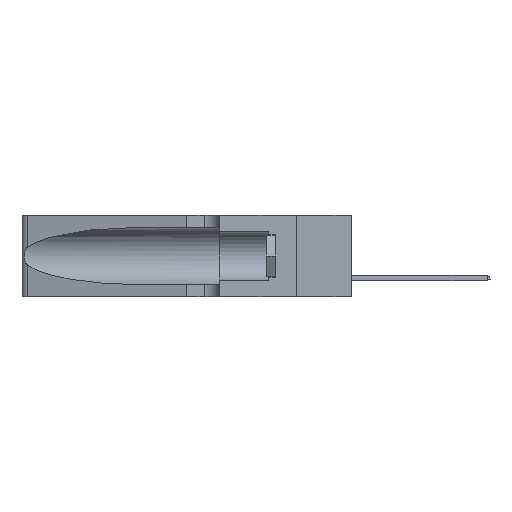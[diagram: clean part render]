
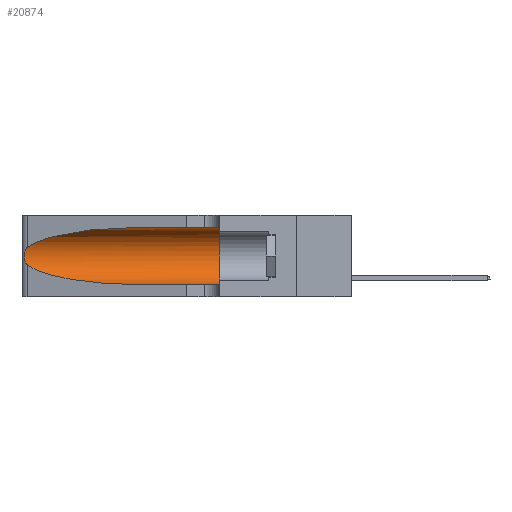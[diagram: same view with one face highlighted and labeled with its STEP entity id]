
A CAD part, left-side view. The second image highlights one B-rep face of the part: STEP entity #20874.
In plain terms, the highlighted cylindrical face has radius 3.308 mm (diameter 6.617 mm), a partial arc.
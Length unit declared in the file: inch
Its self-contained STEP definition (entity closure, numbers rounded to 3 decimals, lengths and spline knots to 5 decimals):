
#215 = CARTESIAN_POINT ( 'NONE',  ( 0.18966, 0.96281, 0.31525 ) ) ;
#1623 = VECTOR ( 'NONE', #15362, 39.37008 ) ;
#1929 = CARTESIAN_POINT ( 'NONE',  ( 0.25487, 1.22718, 0.14631 ) ) ;
#2081 = DIRECTION ( 'NONE',  ( 0., -1., 0. ) ) ;
#2461 = EDGE_CURVE ( 'NONE', #21685, #13691, #21260, .T. ) ;
#2652 = CARTESIAN_POINT ( 'NONE',  ( 0.1305, 0.72297, 0.05475 ) ) ;
#3155 = EDGE_CURVE ( 'NONE', #7632, #14340, #14061, .T. ) ;
#3199 = CARTESIAN_POINT ( 'NONE',  ( 0.25487, 1.22718, 0.14631 ) ) ;
#3279 = EDGE_CURVE ( 'NONE', #3822, #7632, #8387, .T. ) ;
#3552 = CARTESIAN_POINT ( 'NONE',  ( 0.25555, 1.22993, 0.14849 ) ) ;
#3650 = CYLINDRICAL_SURFACE ( 'NONE', #13707, 0.13025 ) ;
#3729 = CARTESIAN_POINT ( 'NONE',  ( 0.25487, 1.22718, 0.14631 ) ) ;
#3822 = VERTEX_POINT ( 'NONE', #19467 ) ;
#3871 = CARTESIAN_POINT ( 'NONE',  ( 0.1305, 0.35, 0.31525 ) ) ;
#4050 = ORIENTED_EDGE ( 'NONE', *, *, #19851, .F. ) ;
#4903 = CARTESIAN_POINT ( 'NONE',  ( 0.18966, 0.96281, 0.05475 ) ) ;
#5049 = CARTESIAN_POINT ( 'NONE',  ( 0.1305, 0.72297, 0.05475 ) ) ;
#5426 = EDGE_LOOP ( 'NONE', ( #5481, #6778, #6812, #5883, #4050, #7863 ) ) ;
#5481 = ORIENTED_EDGE ( 'NONE', *, *, #12679, .T. ) ;
#5562 = CARTESIAN_POINT ( 'NONE',  ( 0.1305, 1.61858, 0.05475 ) ) ;
#5883 = ORIENTED_EDGE ( 'NONE', *, *, #12151, .T. ) ;
#6042 = CARTESIAN_POINT ( 'NONE',  ( 0.1305, 0.72297, 0.31525 ) ) ;
#6211 = CARTESIAN_POINT ( 'NONE',  ( 0.1305, 1.61858, 0.31525 ) ) ;
#6682 = CARTESIAN_POINT ( 'NONE',  ( 0.1305, 0.35, 0.185 ) ) ;
#6778 = ORIENTED_EDGE ( 'NONE', *, *, #3279, .T. ) ;
#6812 = ORIENTED_EDGE ( 'NONE', *, *, #3155, .T. ) ;
#6921 = CARTESIAN_POINT ( 'NONE',  ( 0.25639, 1.23186, 0.15144 ) ) ;
#7130 = CARTESIAN_POINT ( 'NONE',  ( 0.25555, 1.22994, 0.2215 ) ) ;
#7206 = CARTESIAN_POINT ( 'NONE',  ( 0.25789, 1.23486, 0.15765 ) ) ;
#7311 =( BOUNDED_CURVE ( )  B_SPLINE_CURVE ( 3, ( #15368, #215, #17084, #12117 ),
 .UNSPECIFIED., .F., .T. ) 
 B_SPLINE_CURVE_WITH_KNOTS ( ( 4, 4 ),
 ( 1.5708, 2.84003 ),
 .UNSPECIFIED. ) 
 CURVE ( )  GEOMETRIC_REPRESENTATION_ITEM ( )  RATIONAL_B_SPLINE_CURVE ( ( 1., 0.87, 0.87, 1. ) ) 
 REPRESENTATION_ITEM ( '' )  );
#7632 = VERTEX_POINT ( 'NONE', #3729 ) ;
#7863 = ORIENTED_EDGE ( 'NONE', *, *, #2461, .F. ) ;
#8387 = B_SPLINE_CURVE_WITH_KNOTS ( 'NONE', 3,
 ( #17322, #7130, #15400, #20549, #10345, #19030, #12364, #8644, #13765, #10555, #7206, #6921, #3552, #1929 ),
 .UNSPECIFIED., .F., .F.,
 ( 4, 2, 2, 2, 2, 2, 4 ),
 ( 0., 0.00027, 0.00053, 0.00107, 0.0016, 0.00187, 0.00214 ),
 .UNSPECIFIED. ) ;
#8644 = CARTESIAN_POINT ( 'NONE',  ( 0.26075, 1.23896, 0.178 ) ) ;
#9286 = VERTEX_POINT ( 'NONE', #17202 ) ;
#10345 = CARTESIAN_POINT ( 'NONE',  ( 0.25854, 1.2359, 0.20912 ) ) ;
#10555 = CARTESIAN_POINT ( 'NONE',  ( 0.25856, 1.23593, 0.16098 ) ) ;
#11764 = CIRCLE ( 'NONE', #12943, 0.13025 ) ;
#11795 = DIRECTION ( 'NONE',  ( 0., 1., 0. ) ) ;
#12117 = CARTESIAN_POINT ( 'NONE',  ( 0.25487, 1.22718, 0.22369 ) ) ;
#12151 = EDGE_CURVE ( 'NONE', #14340, #9286, #20004, .T. ) ;
#12364 = CARTESIAN_POINT ( 'NONE',  ( 0.26075, 1.23896, 0.19203 ) ) ;
#12679 = EDGE_CURVE ( 'NONE', #21685, #3822, #7311, .T. ) ;
#12943 = AXIS2_PLACEMENT_3D ( 'NONE', #6682, #11795, #14042 ) ;
#13691 = VERTEX_POINT ( 'NONE', #3871 ) ;
#13707 = AXIS2_PLACEMENT_3D ( 'NONE', #15850, #2081, #14552 ) ;
#13765 = CARTESIAN_POINT ( 'NONE',  ( 0.26017, 1.23833, 0.17102 ) ) ;
#13795 = VECTOR ( 'NONE', #15635, 39.37008 ) ;
#14042 = DIRECTION ( 'NONE',  ( 0., 0., 1. ) ) ;
#14061 =( BOUNDED_CURVE ( )  B_SPLINE_CURVE ( 3, ( #3199, #15089, #4903, #5049 ),
 .UNSPECIFIED., .F., .F. ) 
 B_SPLINE_CURVE_WITH_KNOTS ( ( 4, 4 ),
 ( 3.44316, 4.71239 ),
 .UNSPECIFIED. ) 
 CURVE ( )  GEOMETRIC_REPRESENTATION_ITEM ( )  RATIONAL_B_SPLINE_CURVE ( ( 1., 0.87, 0.87, 1. ) ) 
 REPRESENTATION_ITEM ( '' )  );
#14340 = VERTEX_POINT ( 'NONE', #2652 ) ;
#14552 = DIRECTION ( 'NONE',  ( 0., 0., -1. ) ) ;
#15089 = CARTESIAN_POINT ( 'NONE',  ( 0.2373, 1.15595, 0.08982 ) ) ;
#15362 = DIRECTION ( 'NONE',  ( 0., -1., 0. ) ) ;
#15368 = CARTESIAN_POINT ( 'NONE',  ( 0.1305, 0.72297, 0.31525 ) ) ;
#15400 = CARTESIAN_POINT ( 'NONE',  ( 0.25639, 1.23184, 0.21858 ) ) ;
#15635 = DIRECTION ( 'NONE',  ( 0., -1., 0. ) ) ;
#15850 = CARTESIAN_POINT ( 'NONE',  ( 0.1305, 1.61858, 0.185 ) ) ;
#17084 = CARTESIAN_POINT ( 'NONE',  ( 0.2373, 1.15595, 0.28018 ) ) ;
#17202 = CARTESIAN_POINT ( 'NONE',  ( 0.1305, 0.35, 0.05475 ) ) ;
#17322 = CARTESIAN_POINT ( 'NONE',  ( 0.25487, 1.22718, 0.22369 ) ) ;
#19030 = CARTESIAN_POINT ( 'NONE',  ( 0.26018, 1.23835, 0.19895 ) ) ;
#19467 = CARTESIAN_POINT ( 'NONE',  ( 0.25487, 1.22718, 0.22369 ) ) ;
#19851 = EDGE_CURVE ( 'NONE', #13691, #9286, #11764, .T. ) ;
#19953 = FACE_OUTER_BOUND ( 'NONE', #5426, .T. ) ;
#20004 = LINE ( 'NONE', #5562, #1623 ) ;
#20549 = CARTESIAN_POINT ( 'NONE',  ( 0.25787, 1.23484, 0.2124 ) ) ;
#20874 = ADVANCED_FACE ( 'NONE', ( #19953 ), #3650, .F. ) ;
#21260 = LINE ( 'NONE', #6211, #13795 ) ;
#21685 = VERTEX_POINT ( 'NONE', #6042 ) ;
